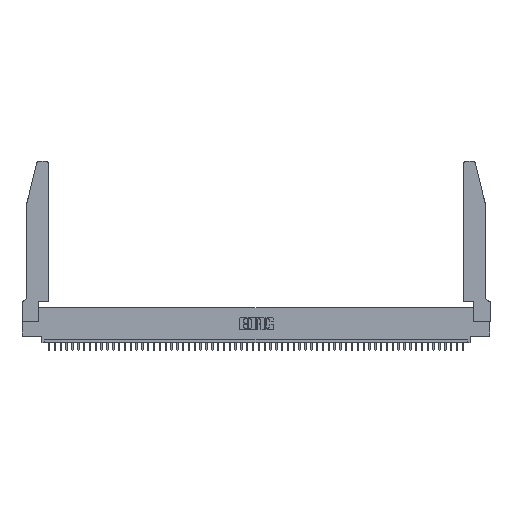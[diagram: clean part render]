
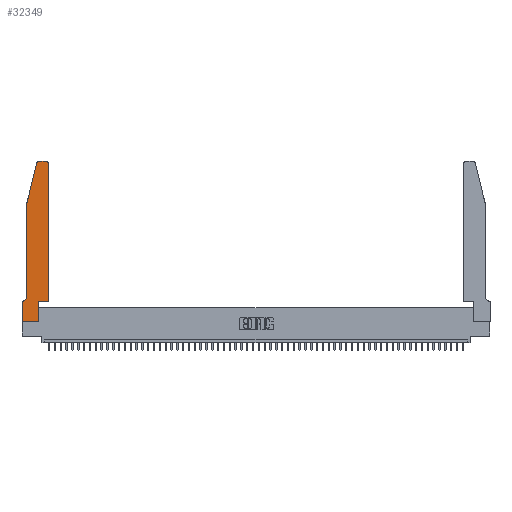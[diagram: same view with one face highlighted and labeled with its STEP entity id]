
A CAD part, top view. The second image highlights one B-rep face of the part: STEP entity #32349.
In plain terms, the highlighted planar face has unit normal (0, 0, 1).
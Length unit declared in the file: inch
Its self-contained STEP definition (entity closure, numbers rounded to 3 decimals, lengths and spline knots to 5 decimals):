
#528 = VECTOR ( 'NONE', #47871, 39.37008 ) ;
#855 = VERTEX_POINT ( 'NONE', #9250 ) ;
#1118 = PLANE ( 'NONE',  #22941 ) ;
#1627 = VERTEX_POINT ( 'NONE', #53356 ) ;
#1788 = VECTOR ( 'NONE', #46687, 39.37008 ) ;
#3350 = ORIENTED_EDGE ( 'NONE', *, *, #48910, .T. ) ;
#3591 = AXIS2_PLACEMENT_3D ( 'NONE', #24385, #50082, #24564 ) ;
#4297 = LINE ( 'NONE', #42179, #21460 ) ;
#4705 = DIRECTION ( 'NONE',  ( 1., 0., 0. ) ) ;
#4972 = VECTOR ( 'NONE', #50557, 39.37008 ) ;
#5786 = LINE ( 'NONE', #16551, #1788 ) ;
#5924 = EDGE_CURVE ( 'NONE', #8222, #15122, #53584, .T. ) ;
#6238 = CARTESIAN_POINT ( 'NONE',  ( 0.0755, 2., 0.37 ) ) ;
#7671 = VECTOR ( 'NONE', #12086, 39.37008 ) ;
#8181 = VERTEX_POINT ( 'NONE', #8611 ) ;
#8222 = VERTEX_POINT ( 'NONE', #34569 ) ;
#8337 = LINE ( 'NONE', #24468, #7671 ) ;
#8611 = CARTESIAN_POINT ( 'NONE',  ( 0., 0.35, 0.37 ) ) ;
#9250 = CARTESIAN_POINT ( 'NONE',  ( 0.2865, 0., 0.37 ) ) ;
#9253 = EDGE_CURVE ( 'NONE', #8181, #21515, #50258, .T. ) ;
#9427 = ORIENTED_EDGE ( 'NONE', *, *, #31792, .T. ) ;
#10158 = VECTOR ( 'NONE', #47752, 39.37008 ) ;
#10975 = ORIENTED_EDGE ( 'NONE', *, *, #51376, .T. ) ;
#11030 = EDGE_CURVE ( 'NONE', #21515, #855, #41698, .T. ) ;
#11759 = CARTESIAN_POINT ( 'NONE',  ( 0., 0., 0.37 ) ) ;
#11997 = ORIENTED_EDGE ( 'NONE', *, *, #41358, .T. ) ;
#12086 = DIRECTION ( 'NONE',  ( 0., 1., 0. ) ) ;
#14555 = DIRECTION ( 'NONE',  ( 0., 1., 0. ) ) ;
#15122 = VERTEX_POINT ( 'NONE', #30504 ) ;
#15174 = CARTESIAN_POINT ( 'NONE',  ( 0.4505, 2.72, 0.37 ) ) ;
#16551 = CARTESIAN_POINT ( 'NONE',  ( 0.2605, 2.75, 0.37 ) ) ;
#17516 = LINE ( 'NONE', #29524, #4972 ) ;
#18640 = DIRECTION ( 'NONE',  ( 0., 0., 1. ) ) ;
#19785 = CARTESIAN_POINT ( 'NONE',  ( 0.25487, 2.72718, 0.37 ) ) ;
#21460 = VECTOR ( 'NONE', #4705, 39.37008 ) ;
#21515 = VERTEX_POINT ( 'NONE', #11759 ) ;
#21580 = AXIS2_PLACEMENT_3D ( 'NONE', #52978, #48687, #48494 ) ;
#22449 = VERTEX_POINT ( 'NONE', #15174 ) ;
#22729 = DIRECTION ( 'NONE',  ( 1., 0., 0. ) ) ;
#22941 = AXIS2_PLACEMENT_3D ( 'NONE', #30584, #18640, #22729 ) ;
#23665 = VERTEX_POINT ( 'NONE', #32079 ) ;
#24385 = CARTESIAN_POINT ( 'NONE',  ( 0.4205, 2.72, 0.37 ) ) ;
#24468 = CARTESIAN_POINT ( 'NONE',  ( 0.2865, 0.35, 0.37 ) ) ;
#24564 = DIRECTION ( 'NONE',  ( 1., 0., 0. ) ) ;
#25237 = VERTEX_POINT ( 'NONE', #42910 ) ;
#26271 = VECTOR ( 'NONE', #31986, 39.37008 ) ;
#27943 = ORIENTED_EDGE ( 'NONE', *, *, #32784, .T. ) ;
#29016 = EDGE_CURVE ( 'NONE', #23665, #8181, #45373, .T. ) ;
#29524 = CARTESIAN_POINT ( 'NONE',  ( 0.0755, 2., 0.37 ) ) ;
#30504 = CARTESIAN_POINT ( 'NONE',  ( 0.0755, 0.42, 0.37 ) ) ;
#30584 = CARTESIAN_POINT ( 'NONE',  ( 0., 0.35, 0.37 ) ) ;
#31250 = CARTESIAN_POINT ( 'NONE',  ( 0.2865, 0.35, 0.37 ) ) ;
#31792 = EDGE_CURVE ( 'NONE', #25237, #46419, #41706, .T. ) ;
#31986 = DIRECTION ( 'NONE',  ( 0., -1., 0. ) ) ;
#32079 = CARTESIAN_POINT ( 'NONE',  ( 0.0055, 0.35, 0.37 ) ) ;
#32349 = ADVANCED_FACE ( 'NONE', ( #41599 ), #1118, .T. ) ;
#32595 = AXIS2_PLACEMENT_3D ( 'NONE', #47941, #36045, #43653 ) ;
#32784 = EDGE_CURVE ( 'NONE', #44090, #22449, #42871, .T. ) ;
#33463 = EDGE_CURVE ( 'NONE', #15122, #23665, #50144, .T. ) ;
#33736 = ORIENTED_EDGE ( 'NONE', *, *, #5924, .T. ) ;
#33948 = CARTESIAN_POINT ( 'NONE',  ( 0.4505, 0.35, 0.37 ) ) ;
#34179 = CARTESIAN_POINT ( 'NONE',  ( 0.0755, 0.35, 0.37 ) ) ;
#34239 = VECTOR ( 'NONE', #14555, 39.37008 ) ;
#34569 = CARTESIAN_POINT ( 'NONE',  ( 0.0755, 2., 0.37 ) ) ;
#36045 = DIRECTION ( 'NONE',  ( 0., 0., 1. ) ) ;
#36902 = ORIENTED_EDGE ( 'NONE', *, *, #49716, .T. ) ;
#37179 = VERTEX_POINT ( 'NONE', #31250 ) ;
#39504 = CARTESIAN_POINT ( 'NONE',  ( 0., 0., 0.37 ) ) ;
#39853 = CARTESIAN_POINT ( 'NONE',  ( 0.4505, 0.35, 0.37 ) ) ;
#40143 = EDGE_CURVE ( 'NONE', #46419, #8222, #17516, .T. ) ;
#40246 = VECTOR ( 'NONE', #43747, 39.37008 ) ;
#41358 = EDGE_CURVE ( 'NONE', #37179, #44090, #4297, .T. ) ;
#41599 = FACE_OUTER_BOUND ( 'NONE', #53533, .T. ) ;
#41698 = LINE ( 'NONE', #39504, #528 ) ;
#41706 = CIRCLE ( 'NONE', #32595, 0.03 ) ;
#42179 = CARTESIAN_POINT ( 'NONE',  ( 0.4505, 0.35, 0.37 ) ) ;
#42871 = LINE ( 'NONE', #39853, #34239 ) ;
#42910 = CARTESIAN_POINT ( 'NONE',  ( 0.284, 2.75, 0.37 ) ) ;
#43653 = DIRECTION ( 'NONE',  ( 1., 0., 0. ) ) ;
#43747 = DIRECTION ( 'NONE',  ( 0., -1., 0. ) ) ;
#44090 = VERTEX_POINT ( 'NONE', #33948 ) ;
#44429 = CIRCLE ( 'NONE', #3591, 0.03 ) ;
#45373 = LINE ( 'NONE', #34179, #10158 ) ;
#46419 = VERTEX_POINT ( 'NONE', #19785 ) ;
#46606 = ORIENTED_EDGE ( 'NONE', *, *, #11030, .T. ) ;
#46687 = DIRECTION ( 'NONE',  ( -1., 0., 0. ) ) ;
#47752 = DIRECTION ( 'NONE',  ( -1., 0., 0. ) ) ;
#47871 = DIRECTION ( 'NONE',  ( 1., 0., 0. ) ) ;
#47941 = CARTESIAN_POINT ( 'NONE',  ( 0.284, 2.72, 0.37 ) ) ;
#48494 = DIRECTION ( 'NONE',  ( -1., 0., 0. ) ) ;
#48570 = CARTESIAN_POINT ( 'NONE',  ( 0., 0., 0.37 ) ) ;
#48687 = DIRECTION ( 'NONE',  ( 0., 0., -1. ) ) ;
#48705 = ORIENTED_EDGE ( 'NONE', *, *, #40143, .T. ) ;
#48910 = EDGE_CURVE ( 'NONE', #22449, #1627, #44429, .T. ) ;
#49716 = EDGE_CURVE ( 'NONE', #1627, #25237, #5786, .T. ) ;
#50082 = DIRECTION ( 'NONE',  ( 0., 0., 1. ) ) ;
#50144 = CIRCLE ( 'NONE', #21580, 0.07 ) ;
#50258 = LINE ( 'NONE', #48570, #40246 ) ;
#50557 = DIRECTION ( 'NONE',  ( -0.239, -0.971, 0. ) ) ;
#50747 = ORIENTED_EDGE ( 'NONE', *, *, #9253, .T. ) ;
#50899 = ORIENTED_EDGE ( 'NONE', *, *, #33463, .T. ) ;
#51376 = EDGE_CURVE ( 'NONE', #855, #37179, #8337, .T. ) ;
#52003 = ORIENTED_EDGE ( 'NONE', *, *, #29016, .T. ) ;
#52978 = CARTESIAN_POINT ( 'NONE',  ( 0.0055, 0.42, 0.37 ) ) ;
#53356 = CARTESIAN_POINT ( 'NONE',  ( 0.4205, 2.75, 0.37 ) ) ;
#53533 = EDGE_LOOP ( 'NONE', ( #36902, #9427, #48705, #33736, #50899, #52003, #50747, #46606, #10975, #11997, #27943, #3350 ) ) ;
#53584 = LINE ( 'NONE', #6238, #26271 ) ;
